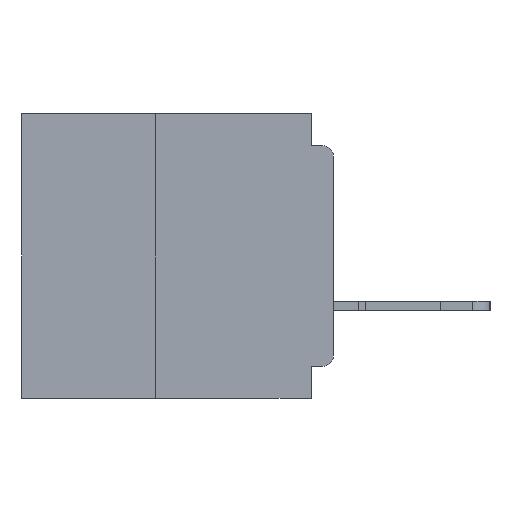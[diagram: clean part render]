
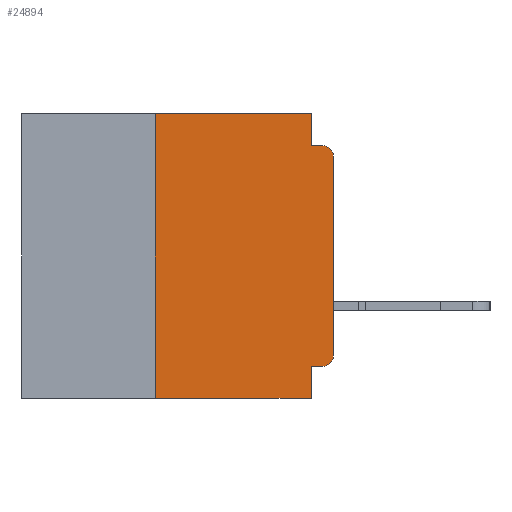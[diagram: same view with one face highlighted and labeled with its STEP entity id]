
A CAD part, left-side view. The second image highlights one B-rep face of the part: STEP entity #24894.
In plain terms, the highlighted planar face has unit normal (-1, 0, 0).
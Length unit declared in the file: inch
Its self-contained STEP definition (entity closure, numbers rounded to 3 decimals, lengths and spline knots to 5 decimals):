
#424 = EDGE_CURVE ( 'NONE', #15972, #37494, #7615, .T. ) ;
#801 = PLANE ( 'NONE',  #51739 ) ;
#1074 = LINE ( 'NONE', #56564, #13875 ) ;
#2207 = CARTESIAN_POINT ( 'NONE',  ( 0., 0., -0.355 ) ) ;
#4040 = DIRECTION ( 'NONE',  ( 0., 0., 1. ) ) ;
#4586 = CARTESIAN_POINT ( 'NONE',  ( 0., 0., -0.06 ) ) ;
#5285 = CARTESIAN_POINT ( 'NONE',  ( 0., 0.031, -0.4 ) ) ;
#5686 = DIRECTION ( 'NONE',  ( 1., 0., 0. ) ) ;
#5893 = VECTOR ( 'NONE', #61950, 39.37008 ) ;
#6076 = ORIENTED_EDGE ( 'NONE', *, *, #61606, .T. ) ;
#6476 = VERTEX_POINT ( 'NONE', #60670 ) ;
#7174 = LINE ( 'NONE', #5285, #31209 ) ;
#7615 = LINE ( 'NONE', #56491, #57023 ) ;
#7670 = ORIENTED_EDGE ( 'NONE', *, *, #8311, .F. ) ;
#8311 = EDGE_CURVE ( 'NONE', #52368, #59888, #1074, .T. ) ;
#11629 = DIRECTION ( 'NONE',  ( 0., -1., 0. ) ) ;
#13875 = VECTOR ( 'NONE', #4040, 39.37008 ) ;
#13907 = CARTESIAN_POINT ( 'NONE',  ( 0., 0.015, -0.06 ) ) ;
#14382 = DIRECTION ( 'NONE',  ( -1., 0., 0. ) ) ;
#15275 = ORIENTED_EDGE ( 'NONE', *, *, #51800, .T. ) ;
#15822 = CARTESIAN_POINT ( 'NONE',  ( 0., 0., -0.34 ) ) ;
#15972 = VERTEX_POINT ( 'NONE', #58111 ) ;
#16689 = EDGE_CURVE ( 'NONE', #51809, #37083, #44713, .T. ) ;
#17859 = VERTEX_POINT ( 'NONE', #39597 ) ;
#18304 = EDGE_CURVE ( 'NONE', #37494, #58155, #56814, .T. ) ;
#18390 = VERTEX_POINT ( 'NONE', #29482 ) ;
#18734 = DIRECTION ( 'NONE',  ( 0., 0., -1. ) ) ;
#18989 = CARTESIAN_POINT ( 'NONE',  ( 0., 0., -0.045 ) ) ;
#19761 = DIRECTION ( 'NONE',  ( 0., 0., -1. ) ) ;
#19960 = ORIENTED_EDGE ( 'NONE', *, *, #16689, .T. ) ;
#20636 = CARTESIAN_POINT ( 'NONE',  ( 0., 0., 0. ) ) ;
#21749 = VECTOR ( 'NONE', #59535, 39.37008 ) ;
#21850 = EDGE_LOOP ( 'NONE', ( #19960, #6076, #59037, #33764, #59437, #7670, #15275, #44286, #52014, #31981 ) ) ;
#23027 = LINE ( 'NONE', #45136, #46932 ) ;
#24894 = ADVANCED_FACE ( 'NONE', ( #35694 ), #801, .F. ) ;
#26531 = AXIS2_PLACEMENT_3D ( 'NONE', #13907, #47404, #18734 ) ;
#28894 = AXIS2_PLACEMENT_3D ( 'NONE', #43096, #14382, #47878 ) ;
#29023 = VECTOR ( 'NONE', #49301, 39.37008 ) ;
#29482 = CARTESIAN_POINT ( 'NONE',  ( 0., 0.031, -0.355 ) ) ;
#30897 = CARTESIAN_POINT ( 'NONE',  ( 0., 0.25, -0.4 ) ) ;
#31209 = VECTOR ( 'NONE', #19761, 39.37008 ) ;
#31981 = ORIENTED_EDGE ( 'NONE', *, *, #51628, .T. ) ;
#32473 = CIRCLE ( 'NONE', #26531, 0.015 ) ;
#33764 = ORIENTED_EDGE ( 'NONE', *, *, #424, .F. ) ;
#34438 = CARTESIAN_POINT ( 'NONE',  ( 0., 0.437, 0. ) ) ;
#34900 = DIRECTION ( 'NONE',  ( 0., -1., 0. ) ) ;
#35694 = FACE_OUTER_BOUND ( 'NONE', #21850, .T. ) ;
#35996 = CARTESIAN_POINT ( 'NONE',  ( 0., 0.031, -0.045 ) ) ;
#37083 = VERTEX_POINT ( 'NONE', #4586 ) ;
#37447 = EDGE_CURVE ( 'NONE', #6476, #18390, #47175, .T. ) ;
#37494 = VERTEX_POINT ( 'NONE', #35996 ) ;
#37672 = CIRCLE ( 'NONE', #28894, 0.015 ) ;
#38386 = LINE ( 'NONE', #58671, #52576 ) ;
#39245 = DIRECTION ( 'NONE',  ( 0., 0., -1. ) ) ;
#39597 = CARTESIAN_POINT ( 'NONE',  ( 0., 0.031, -0.4 ) ) ;
#43096 = CARTESIAN_POINT ( 'NONE',  ( 0., 0.015, -0.34 ) ) ;
#44286 = ORIENTED_EDGE ( 'NONE', *, *, #59992, .F. ) ;
#44713 = LINE ( 'NONE', #20636, #29023 ) ;
#45136 = CARTESIAN_POINT ( 'NONE',  ( 0., 0.437, 0. ) ) ;
#46427 = CARTESIAN_POINT ( 'NONE',  ( 0., 0.015, -0.045 ) ) ;
#46932 = VECTOR ( 'NONE', #11629, 39.37008 ) ;
#47175 = LINE ( 'NONE', #2207, #21749 ) ;
#47404 = DIRECTION ( 'NONE',  ( -1., 0., 0. ) ) ;
#47878 = DIRECTION ( 'NONE',  ( 0., 0., -1. ) ) ;
#49301 = DIRECTION ( 'NONE',  ( 0., 0., 1. ) ) ;
#51628 = EDGE_CURVE ( 'NONE', #6476, #51809, #37672, .T. ) ;
#51739 = AXIS2_PLACEMENT_3D ( 'NONE', #34438, #5686, #39245 ) ;
#51800 = EDGE_CURVE ( 'NONE', #52368, #17859, #38386, .T. ) ;
#51809 = VERTEX_POINT ( 'NONE', #15822 ) ;
#52014 = ORIENTED_EDGE ( 'NONE', *, *, #37447, .F. ) ;
#52368 = VERTEX_POINT ( 'NONE', #30897 ) ;
#52430 = CARTESIAN_POINT ( 'NONE',  ( 0., 0.25, 0. ) ) ;
#52576 = VECTOR ( 'NONE', #34900, 39.37008 ) ;
#55553 = DIRECTION ( 'NONE',  ( 0., 0., -1. ) ) ;
#56491 = CARTESIAN_POINT ( 'NONE',  ( 0., 0.031, 0. ) ) ;
#56564 = CARTESIAN_POINT ( 'NONE',  ( 0., 0.25, -0.4 ) ) ;
#56814 = LINE ( 'NONE', #18989, #5893 ) ;
#57023 = VECTOR ( 'NONE', #55553, 39.37008 ) ;
#58111 = CARTESIAN_POINT ( 'NONE',  ( 0., 0.031, 0. ) ) ;
#58155 = VERTEX_POINT ( 'NONE', #46427 ) ;
#58671 = CARTESIAN_POINT ( 'NONE',  ( 0., 0.437, -0.4 ) ) ;
#59037 = ORIENTED_EDGE ( 'NONE', *, *, #18304, .F. ) ;
#59437 = ORIENTED_EDGE ( 'NONE', *, *, #59543, .F. ) ;
#59535 = DIRECTION ( 'NONE',  ( 0., 1., 0. ) ) ;
#59543 = EDGE_CURVE ( 'NONE', #59888, #15972, #23027, .T. ) ;
#59888 = VERTEX_POINT ( 'NONE', #52430 ) ;
#59992 = EDGE_CURVE ( 'NONE', #18390, #17859, #7174, .T. ) ;
#60670 = CARTESIAN_POINT ( 'NONE',  ( 0., 0.015, -0.355 ) ) ;
#61606 = EDGE_CURVE ( 'NONE', #37083, #58155, #32473, .T. ) ;
#61950 = DIRECTION ( 'NONE',  ( 0., -1., 0. ) ) ;
